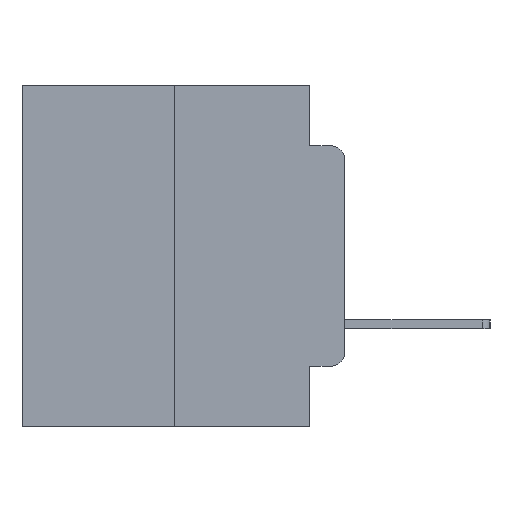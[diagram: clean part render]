
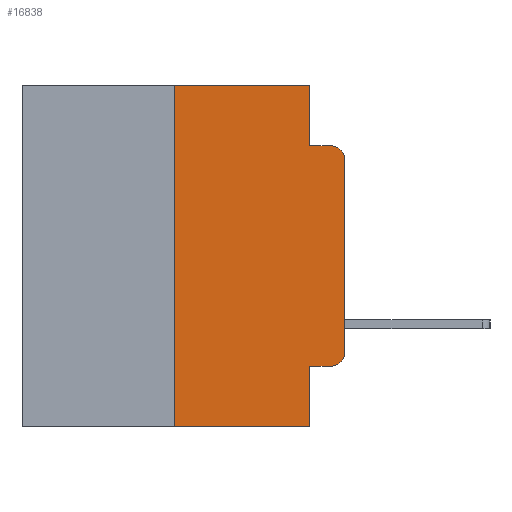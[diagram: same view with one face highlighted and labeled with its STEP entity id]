
A CAD part, left-side view. The second image highlights one B-rep face of the part: STEP entity #16838.
In plain terms, the highlighted planar face has unit normal (-1, 0, 0).
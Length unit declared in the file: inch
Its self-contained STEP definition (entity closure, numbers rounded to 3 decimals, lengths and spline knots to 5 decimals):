
#248 = LINE ( 'NONE', #14994, #16080 ) ;
#403 = VERTEX_POINT ( 'NONE', #20564 ) ;
#738 = EDGE_CURVE ( 'NONE', #4007, #9798, #18041, .T. ) ;
#1237 = ORIENTED_EDGE ( 'NONE', *, *, #17515, .T. ) ;
#1493 = VERTEX_POINT ( 'NONE', #13708 ) ;
#2642 = EDGE_CURVE ( 'NONE', #7757, #5245, #6570, .T. ) ;
#2936 = AXIS2_PLACEMENT_3D ( 'NONE', #4292, #18533, #6421 ) ;
#4007 = VERTEX_POINT ( 'NONE', #9478 ) ;
#4207 = ORIENTED_EDGE ( 'NONE', *, *, #15153, .F. ) ;
#4274 = LINE ( 'NONE', #21178, #14608 ) ;
#4292 = CARTESIAN_POINT ( 'NONE',  ( 0., 0.02, -0.1085 ) ) ;
#4356 = CARTESIAN_POINT ( 'NONE',  ( 0., 0.051, 0. ) ) ;
#4560 = CIRCLE ( 'NONE', #2936, 0.02 ) ;
#4565 = VECTOR ( 'NONE', #19373, 39.37008 ) ;
#4924 = PLANE ( 'NONE',  #14904 ) ;
#5245 = VERTEX_POINT ( 'NONE', #6192 ) ;
#5645 = DIRECTION ( 'NONE',  ( 0., 0., 1. ) ) ;
#6139 = AXIS2_PLACEMENT_3D ( 'NONE', #23392, #11706, #25279 ) ;
#6192 = CARTESIAN_POINT ( 'NONE',  ( 0., 0.051, -0.5 ) ) ;
#6263 = DIRECTION ( 'NONE',  ( 0., 0., -1. ) ) ;
#6348 = EDGE_LOOP ( 'NONE', ( #7858, #18539, #13878, #4207, #21507, #22105, #1237, #17661, #8214, #10187 ) ) ;
#6421 = DIRECTION ( 'NONE',  ( 0., 0., -1. ) ) ;
#6536 = LINE ( 'NONE', #13998, #16112 ) ;
#6570 = LINE ( 'NONE', #17316, #4565 ) ;
#7082 = DIRECTION ( 'NONE',  ( 0., 0., -1. ) ) ;
#7345 = LINE ( 'NONE', #18387, #14301 ) ;
#7757 = VERTEX_POINT ( 'NONE', #9133 ) ;
#7858 = ORIENTED_EDGE ( 'NONE', *, *, #738, .T. ) ;
#7884 = CARTESIAN_POINT ( 'NONE',  ( 0., 0.051, -0.0885 ) ) ;
#8214 = ORIENTED_EDGE ( 'NONE', *, *, #23336, .T. ) ;
#8367 = EDGE_CURVE ( 'NONE', #9634, #15197, #8755, .T. ) ;
#8593 = CARTESIAN_POINT ( 'NONE',  ( 0., 0.02, -0.4115 ) ) ;
#8755 = LINE ( 'NONE', #17838, #14075 ) ;
#9133 = CARTESIAN_POINT ( 'NONE',  ( 0., 0.051, -0.4115 ) ) ;
#9478 = CARTESIAN_POINT ( 'NONE',  ( 0., 0., -0.3915 ) ) ;
#9634 = VERTEX_POINT ( 'NONE', #21849 ) ;
#9798 = VERTEX_POINT ( 'NONE', #10800 ) ;
#10187 = ORIENTED_EDGE ( 'NONE', *, *, #17003, .T. ) ;
#10800 = CARTESIAN_POINT ( 'NONE',  ( 0., 0., -0.1085 ) ) ;
#11706 = DIRECTION ( 'NONE',  ( -1., 0., 0. ) ) ;
#12536 = CARTESIAN_POINT ( 'NONE',  ( 0., 0.25, 0. ) ) ;
#12738 = VECTOR ( 'NONE', #23805, 39.37008 ) ;
#13708 = CARTESIAN_POINT ( 'NONE',  ( 0., 0.02, -0.0885 ) ) ;
#13878 = ORIENTED_EDGE ( 'NONE', *, *, #17791, .F. ) ;
#13998 = CARTESIAN_POINT ( 'NONE',  ( 0., 0.051, -0.4115 ) ) ;
#14075 = VECTOR ( 'NONE', #5645, 39.37008 ) ;
#14301 = VECTOR ( 'NONE', #6263, 39.37008 ) ;
#14608 = VECTOR ( 'NONE', #23068, 39.37008 ) ;
#14904 = AXIS2_PLACEMENT_3D ( 'NONE', #24732, #19105, #7082 ) ;
#14994 = CARTESIAN_POINT ( 'NONE',  ( 0., 0.473, -0.5 ) ) ;
#15153 = EDGE_CURVE ( 'NONE', #21574, #403, #7345, .T. ) ;
#15197 = VERTEX_POINT ( 'NONE', #12536 ) ;
#16080 = VECTOR ( 'NONE', #18922, 39.37008 ) ;
#16112 = VECTOR ( 'NONE', #23306, 39.37008 ) ;
#16838 = ADVANCED_FACE ( 'NONE', ( #20330 ), #4924, .F. ) ;
#17003 = EDGE_CURVE ( 'NONE', #18574, #4007, #21794, .T. ) ;
#17316 = CARTESIAN_POINT ( 'NONE',  ( 0., 0.051, 0. ) ) ;
#17515 = EDGE_CURVE ( 'NONE', #9634, #5245, #248, .T. ) ;
#17661 = ORIENTED_EDGE ( 'NONE', *, *, #2642, .F. ) ;
#17791 = EDGE_CURVE ( 'NONE', #403, #1493, #25858, .T. ) ;
#17838 = CARTESIAN_POINT ( 'NONE',  ( 0., 0.25, 0. ) ) ;
#17996 = DIRECTION ( 'NONE',  ( 0., -1., 0. ) ) ;
#18041 = LINE ( 'NONE', #24415, #12738 ) ;
#18387 = CARTESIAN_POINT ( 'NONE',  ( 0., 0.051, 0. ) ) ;
#18533 = DIRECTION ( 'NONE',  ( -1., 0., 0. ) ) ;
#18539 = ORIENTED_EDGE ( 'NONE', *, *, #22865, .T. ) ;
#18574 = VERTEX_POINT ( 'NONE', #8593 ) ;
#18922 = DIRECTION ( 'NONE',  ( 0., -1., 0. ) ) ;
#19105 = DIRECTION ( 'NONE',  ( 1., 0., 0. ) ) ;
#19373 = DIRECTION ( 'NONE',  ( 0., 0., -1. ) ) ;
#20330 = FACE_OUTER_BOUND ( 'NONE', #6348, .T. ) ;
#20564 = CARTESIAN_POINT ( 'NONE',  ( 0., 0.051, -0.0885 ) ) ;
#20881 = VECTOR ( 'NONE', #17996, 39.37008 ) ;
#21028 = EDGE_CURVE ( 'NONE', #15197, #21574, #4274, .T. ) ;
#21178 = CARTESIAN_POINT ( 'NONE',  ( 0., 0.473, 0. ) ) ;
#21507 = ORIENTED_EDGE ( 'NONE', *, *, #21028, .F. ) ;
#21574 = VERTEX_POINT ( 'NONE', #4356 ) ;
#21794 = CIRCLE ( 'NONE', #6139, 0.02 ) ;
#21849 = CARTESIAN_POINT ( 'NONE',  ( 0., 0.25, -0.5 ) ) ;
#22105 = ORIENTED_EDGE ( 'NONE', *, *, #8367, .F. ) ;
#22865 = EDGE_CURVE ( 'NONE', #9798, #1493, #4560, .T. ) ;
#23068 = DIRECTION ( 'NONE',  ( 0., -1., 0. ) ) ;
#23306 = DIRECTION ( 'NONE',  ( 0., -1., 0. ) ) ;
#23336 = EDGE_CURVE ( 'NONE', #7757, #18574, #6536, .T. ) ;
#23392 = CARTESIAN_POINT ( 'NONE',  ( 0., 0.02, -0.3915 ) ) ;
#23805 = DIRECTION ( 'NONE',  ( 0., 0., 1. ) ) ;
#24415 = CARTESIAN_POINT ( 'NONE',  ( 0., 0., 0. ) ) ;
#24732 = CARTESIAN_POINT ( 'NONE',  ( 0., 0.473, 0. ) ) ;
#25279 = DIRECTION ( 'NONE',  ( 0., 0., -1. ) ) ;
#25858 = LINE ( 'NONE', #7884, #20881 ) ;
